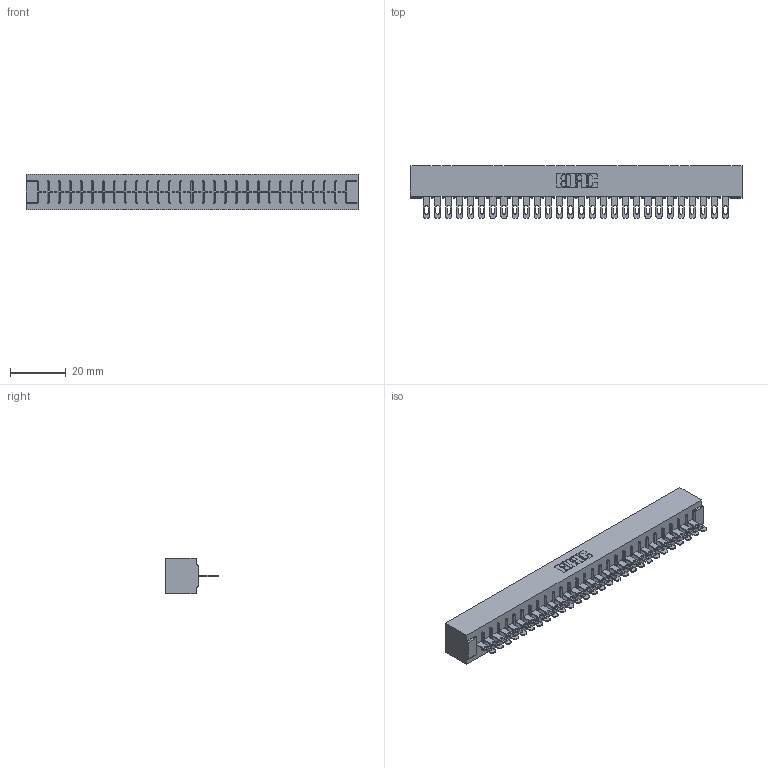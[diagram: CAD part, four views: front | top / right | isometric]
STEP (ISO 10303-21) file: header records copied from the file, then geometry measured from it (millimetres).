
FILE_DESCRIPTION (( 'STEP AP203' ), '1' );
FILE_NAME ('316-028-500-101.STEP', '2018-07-31T02:50:52', ( '' ), ( '' ), 'SwSTEP 2.0', 'SolidWorks 2016', '' );
FILE_SCHEMA (( 'CONFIG_CONTROL_DESIGN' ));
Length unit declared in the file: inch
Products named in the file (3): 306 Part_No Mounting; 306-290-001_100; 316-028-500-101
Assembly tree (29 placements, depth 2):
  316-028-500-101
    306 Part_No Mounting
    306-290-001_100  x28
Bounding box: 118.82 x 18.87 x 12.7 mm (x, y, z)
Volume: 13686.8 mm3; surface area: 14520.5 mm2
Topology: 29 solids, 29 shells, 2236 faces, 6312 edges, 4056 vertices
Faces by surface type: plane 1464, cylinder 660, sphere 112
Entity records: 27811 total; most frequent: CARTESIAN_POINT 4667, ORIENTED_EDGE 4624, DIRECTION 4604, EDGE_CURVE 2312, VECTOR 1802, LINE 1802, VERTEX_POINT 1464, AXIS2_PLACEMENT_3D 1401
